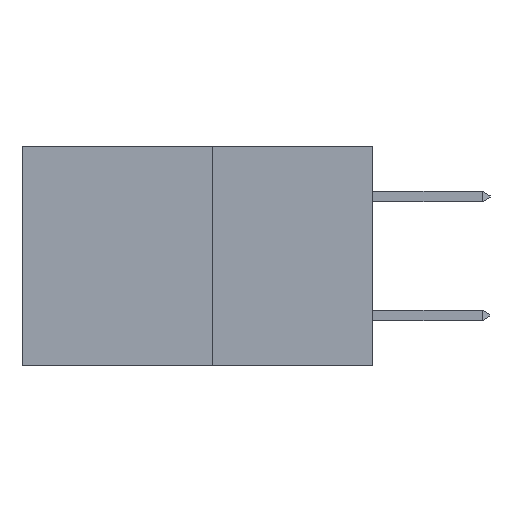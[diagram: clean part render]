
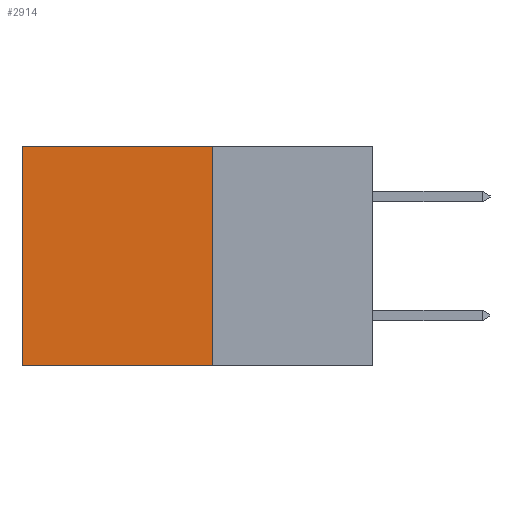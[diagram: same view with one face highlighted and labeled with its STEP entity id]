
A CAD part, left-side view. The second image highlights one B-rep face of the part: STEP entity #2914.
In plain terms, the highlighted planar face has unit normal (-1, 0, 0).
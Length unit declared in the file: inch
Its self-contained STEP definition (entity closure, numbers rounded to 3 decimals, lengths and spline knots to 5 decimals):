
#892 = DIRECTION ( 'NONE',  ( 0., 0., -1. ) ) ;
#918 = ORIENTED_EDGE ( 'NONE', *, *, #6277, .T. ) ;
#1275 = DIRECTION ( 'NONE',  ( 0., 1., 0. ) ) ;
#1359 = CARTESIAN_POINT ( 'NONE',  ( 0.277, 0.27, 0. ) ) ;
#1757 = VERTEX_POINT ( 'NONE', #6978 ) ;
#1956 = LINE ( 'NONE', #2668, #13745 ) ;
#2080 = CARTESIAN_POINT ( 'NONE',  ( 0.277, 0.27, -0.37 ) ) ;
#2173 = ORIENTED_EDGE ( 'NONE', *, *, #14291, .F. ) ;
#2668 = CARTESIAN_POINT ( 'NONE',  ( 0.277, 0.27, -0.37 ) ) ;
#2774 = LINE ( 'NONE', #1359, #8461 ) ;
#2914 = ADVANCED_FACE ( 'NONE', ( #6374 ), #13548, .F. ) ;
#3173 = CARTESIAN_POINT ( 'NONE',  ( 0.277, 0.27, 0. ) ) ;
#3686 = DIRECTION ( 'NONE',  ( 0., 1., 0. ) ) ;
#3787 = DIRECTION ( 'NONE',  ( 0., 0., -1. ) ) ;
#5367 = CARTESIAN_POINT ( 'NONE',  ( 0.277, 0.59, 0. ) ) ;
#5622 = LINE ( 'NONE', #5873, #11456 ) ;
#5873 = CARTESIAN_POINT ( 'NONE',  ( 0.277, 0.27, -0.37 ) ) ;
#6139 = VERTEX_POINT ( 'NONE', #3173 ) ;
#6277 = EDGE_CURVE ( 'NONE', #6139, #14676, #2774, .T. ) ;
#6374 = FACE_OUTER_BOUND ( 'NONE', #11186, .T. ) ;
#6690 = VECTOR ( 'NONE', #892, 39.37008 ) ;
#6978 = CARTESIAN_POINT ( 'NONE',  ( 0.277, 0.59, -0.37 ) ) ;
#7292 = VERTEX_POINT ( 'NONE', #8649 ) ;
#7306 = ORIENTED_EDGE ( 'NONE', *, *, #14641, .T. ) ;
#8461 = VECTOR ( 'NONE', #1275, 39.37008 ) ;
#8649 = CARTESIAN_POINT ( 'NONE',  ( 0.277, 0.27, -0.37 ) ) ;
#9787 = LINE ( 'NONE', #14571, #6690 ) ;
#9979 = DIRECTION ( 'NONE',  ( 0., 0., -1. ) ) ;
#11186 = EDGE_LOOP ( 'NONE', ( #7306, #2173, #12406, #918 ) ) ;
#11259 = AXIS2_PLACEMENT_3D ( 'NONE', #2080, #13665, #9979 ) ;
#11456 = VECTOR ( 'NONE', #3686, 39.37008 ) ;
#12406 = ORIENTED_EDGE ( 'NONE', *, *, #14337, .F. ) ;
#13548 = PLANE ( 'NONE',  #11259 ) ;
#13665 = DIRECTION ( 'NONE',  ( 1., 0., 0. ) ) ;
#13745 = VECTOR ( 'NONE', #3787, 39.37008 ) ;
#14291 = EDGE_CURVE ( 'NONE', #7292, #1757, #5622, .T. ) ;
#14337 = EDGE_CURVE ( 'NONE', #6139, #7292, #1956, .T. ) ;
#14571 = CARTESIAN_POINT ( 'NONE',  ( 0.277, 0.59, -0.37 ) ) ;
#14641 = EDGE_CURVE ( 'NONE', #14676, #1757, #9787, .T. ) ;
#14676 = VERTEX_POINT ( 'NONE', #5367 ) ;
